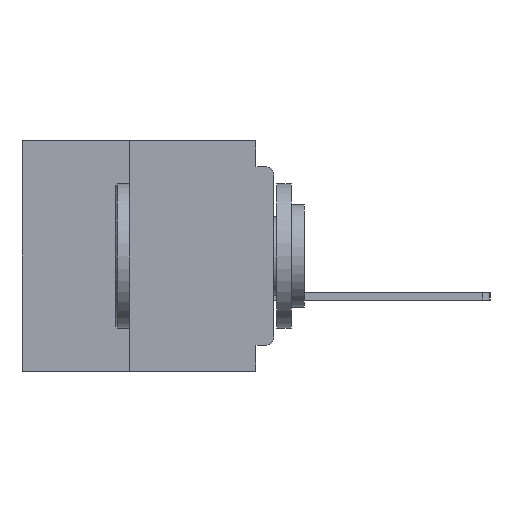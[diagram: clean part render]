
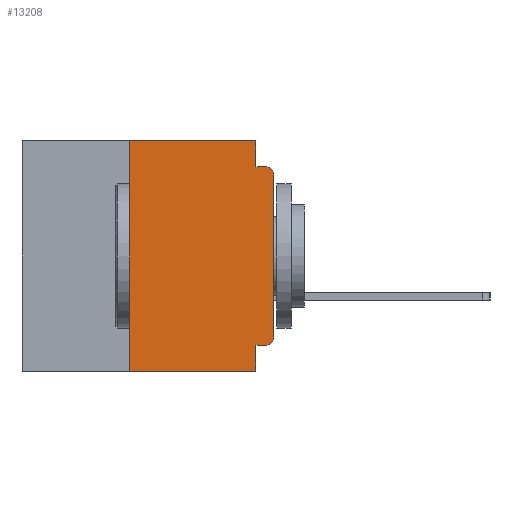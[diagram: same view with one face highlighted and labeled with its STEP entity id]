
A CAD part, left-side view. The second image highlights one B-rep face of the part: STEP entity #13208.
In plain terms, the highlighted planar face has unit normal (-1, 0, 0).
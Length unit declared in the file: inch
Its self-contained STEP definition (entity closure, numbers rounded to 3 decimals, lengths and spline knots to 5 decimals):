
#49 = EDGE_CURVE ( 'NONE', #8089, #21180, #15461, .T. ) ;
#513 = CARTESIAN_POINT ( 'NONE',  ( 0., 0.031, 0. ) ) ;
#746 = DIRECTION ( 'NONE',  ( 0., 0., 1. ) ) ;
#878 = CARTESIAN_POINT ( 'NONE',  ( 0., 0., 0. ) ) ;
#963 = CIRCLE ( 'NONE', #16297, 0.015 ) ;
#1146 = VERTEX_POINT ( 'NONE', #41745 ) ;
#1215 = ORIENTED_EDGE ( 'NONE', *, *, #6080, .F. ) ;
#2021 = DIRECTION ( 'NONE',  ( -1., 0., 0. ) ) ;
#2426 = DIRECTION ( 'NONE',  ( 0., -1., 0. ) ) ;
#2766 = VECTOR ( 'NONE', #5396, 39.37008 ) ;
#3650 = EDGE_CURVE ( 'NONE', #7999, #15208, #15837, .T. ) ;
#4442 = CARTESIAN_POINT ( 'NONE',  ( 0., 0., -0.045 ) ) ;
#4471 = DIRECTION ( 'NONE',  ( 1., 0., 0. ) ) ;
#5396 = DIRECTION ( 'NONE',  ( 0., -1., 0. ) ) ;
#6080 = EDGE_CURVE ( 'NONE', #9259, #31915, #42086, .T. ) ;
#7280 = LINE ( 'NONE', #16373, #16167 ) ;
#7999 = VERTEX_POINT ( 'NONE', #31233 ) ;
#8089 = VERTEX_POINT ( 'NONE', #18199 ) ;
#8815 = CARTESIAN_POINT ( 'NONE',  ( 0., 0.437, -0.4 ) ) ;
#9181 = ORIENTED_EDGE ( 'NONE', *, *, #9280, .T. ) ;
#9251 = DIRECTION ( 'NONE',  ( 0., 0., -1. ) ) ;
#9259 = VERTEX_POINT ( 'NONE', #27922 ) ;
#9280 = EDGE_CURVE ( 'NONE', #9259, #7999, #963, .T. ) ;
#9730 = LINE ( 'NONE', #35828, #42872 ) ;
#10834 = DIRECTION ( 'NONE',  ( 0., -1., 0. ) ) ;
#11854 = LINE ( 'NONE', #8815, #2766 ) ;
#12134 = CARTESIAN_POINT ( 'NONE',  ( 0., 0., -0.355 ) ) ;
#12486 = ORIENTED_EDGE ( 'NONE', *, *, #32780, .T. ) ;
#12494 = EDGE_CURVE ( 'NONE', #32809, #33841, #31055, .T. ) ;
#13208 = ADVANCED_FACE ( 'NONE', ( #21170 ), #37701, .F. ) ;
#13651 = AXIS2_PLACEMENT_3D ( 'NONE', #31027, #4471, #27814 ) ;
#15208 = VERTEX_POINT ( 'NONE', #15477 ) ;
#15461 = LINE ( 'NONE', #4442, #23246 ) ;
#15477 = CARTESIAN_POINT ( 'NONE',  ( 0., 0., -0.06 ) ) ;
#15837 = LINE ( 'NONE', #878, #23613 ) ;
#16111 = EDGE_CURVE ( 'NONE', #15208, #21180, #40527, .T. ) ;
#16167 = VECTOR ( 'NONE', #39259, 39.37008 ) ;
#16297 = AXIS2_PLACEMENT_3D ( 'NONE', #18820, #41946, #22128 ) ;
#16373 = CARTESIAN_POINT ( 'NONE',  ( 0., 0.031, -0.4 ) ) ;
#16610 = VECTOR ( 'NONE', #746, 39.37008 ) ;
#16642 = EDGE_LOOP ( 'NONE', ( #37815, #21319, #37396, #27123, #33639, #25295, #12486, #25110, #1215, #9181 ) ) ;
#17149 = EDGE_CURVE ( 'NONE', #1146, #32809, #25428, .T. ) ;
#17752 = CARTESIAN_POINT ( 'NONE',  ( 0., 0.031, -0.4 ) ) ;
#18199 = CARTESIAN_POINT ( 'NONE',  ( 0., 0.031, -0.045 ) ) ;
#18820 = CARTESIAN_POINT ( 'NONE',  ( 0., 0.015, -0.34 ) ) ;
#18872 = CARTESIAN_POINT ( 'NONE',  ( 0., 0.25, 0. ) ) ;
#20354 = CARTESIAN_POINT ( 'NONE',  ( 0., 0.031, -0.355 ) ) ;
#20681 = CARTESIAN_POINT ( 'NONE',  ( 0., 0.437, 0. ) ) ;
#20885 = CARTESIAN_POINT ( 'NONE',  ( 0., 0.25, -0.4 ) ) ;
#21170 = FACE_OUTER_BOUND ( 'NONE', #16642, .T. ) ;
#21180 = VERTEX_POINT ( 'NONE', #37727 ) ;
#21319 = ORIENTED_EDGE ( 'NONE', *, *, #16111, .T. ) ;
#22128 = DIRECTION ( 'NONE',  ( 0., 0., -1. ) ) ;
#22129 = CARTESIAN_POINT ( 'NONE',  ( 0., 0.015, -0.06 ) ) ;
#23246 = VECTOR ( 'NONE', #2426, 39.37008 ) ;
#23613 = VECTOR ( 'NONE', #35993, 39.37008 ) ;
#25110 = ORIENTED_EDGE ( 'NONE', *, *, #25330, .F. ) ;
#25295 = ORIENTED_EDGE ( 'NONE', *, *, #17149, .F. ) ;
#25330 = EDGE_CURVE ( 'NONE', #31915, #30375, #7280, .T. ) ;
#25428 = LINE ( 'NONE', #20885, #16610 ) ;
#25477 = DIRECTION ( 'NONE',  ( 0., 0., -1. ) ) ;
#27123 = ORIENTED_EDGE ( 'NONE', *, *, #32885, .F. ) ;
#27814 = DIRECTION ( 'NONE',  ( 0., 0., -1. ) ) ;
#27922 = CARTESIAN_POINT ( 'NONE',  ( 0., 0.015, -0.355 ) ) ;
#29784 = AXIS2_PLACEMENT_3D ( 'NONE', #22129, #2021, #25477 ) ;
#30375 = VERTEX_POINT ( 'NONE', #17752 ) ;
#31027 = CARTESIAN_POINT ( 'NONE',  ( 0., 0.437, 0. ) ) ;
#31055 = LINE ( 'NONE', #20681, #38821 ) ;
#31233 = CARTESIAN_POINT ( 'NONE',  ( 0., 0., -0.34 ) ) ;
#31915 = VERTEX_POINT ( 'NONE', #20354 ) ;
#32780 = EDGE_CURVE ( 'NONE', #1146, #30375, #11854, .T. ) ;
#32809 = VERTEX_POINT ( 'NONE', #18872 ) ;
#32885 = EDGE_CURVE ( 'NONE', #33841, #8089, #9730, .T. ) ;
#33639 = ORIENTED_EDGE ( 'NONE', *, *, #12494, .F. ) ;
#33841 = VERTEX_POINT ( 'NONE', #513 ) ;
#35828 = CARTESIAN_POINT ( 'NONE',  ( 0., 0.031, 0. ) ) ;
#35993 = DIRECTION ( 'NONE',  ( 0., 0., 1. ) ) ;
#37396 = ORIENTED_EDGE ( 'NONE', *, *, #49, .F. ) ;
#37701 = PLANE ( 'NONE',  #13651 ) ;
#37727 = CARTESIAN_POINT ( 'NONE',  ( 0., 0.015, -0.045 ) ) ;
#37815 = ORIENTED_EDGE ( 'NONE', *, *, #3650, .T. ) ;
#38821 = VECTOR ( 'NONE', #10834, 39.37008 ) ;
#39259 = DIRECTION ( 'NONE',  ( 0., 0., -1. ) ) ;
#40527 = CIRCLE ( 'NONE', #29784, 0.015 ) ;
#41066 = VECTOR ( 'NONE', #41915, 39.37008 ) ;
#41745 = CARTESIAN_POINT ( 'NONE',  ( 0., 0.25, -0.4 ) ) ;
#41915 = DIRECTION ( 'NONE',  ( 0., 1., 0. ) ) ;
#41946 = DIRECTION ( 'NONE',  ( -1., 0., 0. ) ) ;
#42086 = LINE ( 'NONE', #12134, #41066 ) ;
#42872 = VECTOR ( 'NONE', #9251, 39.37008 ) ;
